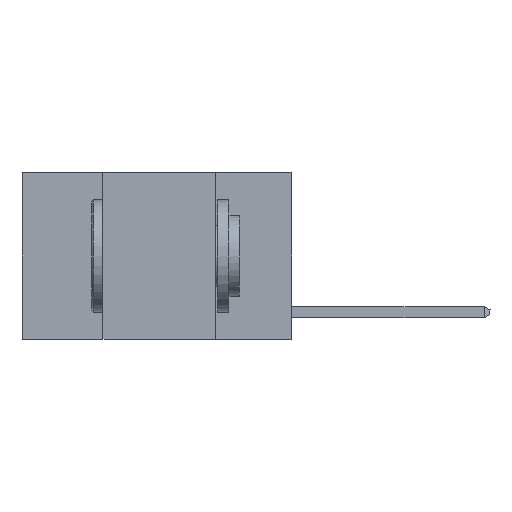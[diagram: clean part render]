
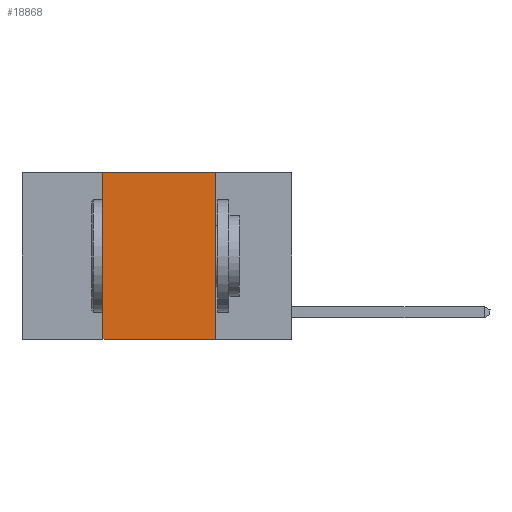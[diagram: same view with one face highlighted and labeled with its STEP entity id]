
A CAD part, left-side view. The second image highlights one B-rep face of the part: STEP entity #18868.
In plain terms, the highlighted planar face has unit normal (-1, 0, 0).
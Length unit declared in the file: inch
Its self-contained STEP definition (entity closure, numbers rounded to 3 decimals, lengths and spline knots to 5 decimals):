
#637 = CARTESIAN_POINT ( 'NONE',  ( 0., 0.6, -0.37 ) ) ;
#669 = CARTESIAN_POINT ( 'NONE',  ( 0., 0.42, 0. ) ) ;
#674 = CARTESIAN_POINT ( 'NONE',  ( 0., 0.17, 0. ) ) ;
#850 = CARTESIAN_POINT ( 'NONE',  ( 0., 0.17, 0. ) ) ;
#1500 = EDGE_CURVE ( 'NONE', #6824, #15678, #15296, .T. ) ;
#1580 = EDGE_LOOP ( 'NONE', ( #11149, #12529, #12674, #6669 ) ) ;
#1696 = CARTESIAN_POINT ( 'NONE',  ( 0., 0.42, -0.37 ) ) ;
#2498 = VECTOR ( 'NONE', #13580, 39.37008 ) ;
#2579 = LINE ( 'NONE', #850, #8392 ) ;
#3430 = VERTEX_POINT ( 'NONE', #674 ) ;
#4036 = CARTESIAN_POINT ( 'NONE',  ( 0., 0.6, 0. ) ) ;
#4053 = EDGE_CURVE ( 'NONE', #3430, #16246, #2579, .T. ) ;
#4987 = DIRECTION ( 'NONE',  ( 1., 0., 0. ) ) ;
#5535 = EDGE_CURVE ( 'NONE', #15678, #3430, #7504, .T. ) ;
#6535 = FACE_OUTER_BOUND ( 'NONE', #1580, .T. ) ;
#6669 = ORIENTED_EDGE ( 'NONE', *, *, #13498, .T. ) ;
#6824 = VERTEX_POINT ( 'NONE', #1696 ) ;
#7246 = CARTESIAN_POINT ( 'NONE',  ( 0., 0.42, 0. ) ) ;
#7504 = LINE ( 'NONE', #4036, #12402 ) ;
#8392 = VECTOR ( 'NONE', #17758, 39.37008 ) ;
#9866 = DIRECTION ( 'NONE',  ( 0., -1., 0. ) ) ;
#11149 = ORIENTED_EDGE ( 'NONE', *, *, #4053, .F. ) ;
#11163 = DIRECTION ( 'NONE',  ( 0., 0., -1. ) ) ;
#11335 = CARTESIAN_POINT ( 'NONE',  ( 0., 0.17, -0.37 ) ) ;
#12402 = VECTOR ( 'NONE', #19718, 39.37008 ) ;
#12529 = ORIENTED_EDGE ( 'NONE', *, *, #5535, .F. ) ;
#12663 = PLANE ( 'NONE',  #17692 ) ;
#12674 = ORIENTED_EDGE ( 'NONE', *, *, #1500, .F. ) ;
#13498 = EDGE_CURVE ( 'NONE', #6824, #16246, #19150, .T. ) ;
#13580 = DIRECTION ( 'NONE',  ( 0., 0., 1. ) ) ;
#15296 = LINE ( 'NONE', #7246, #2498 ) ;
#15678 = VERTEX_POINT ( 'NONE', #669 ) ;
#16246 = VERTEX_POINT ( 'NONE', #11335 ) ;
#17692 = AXIS2_PLACEMENT_3D ( 'NONE', #18835, #4987, #11163 ) ;
#17758 = DIRECTION ( 'NONE',  ( 0., 0., -1. ) ) ;
#18069 = VECTOR ( 'NONE', #9866, 39.37008 ) ;
#18835 = CARTESIAN_POINT ( 'NONE',  ( 0., 0.6, 0. ) ) ;
#18868 = ADVANCED_FACE ( 'NONE', ( #6535 ), #12663, .F. ) ;
#19150 = LINE ( 'NONE', #637, #18069 ) ;
#19718 = DIRECTION ( 'NONE',  ( 0., -1., 0. ) ) ;
